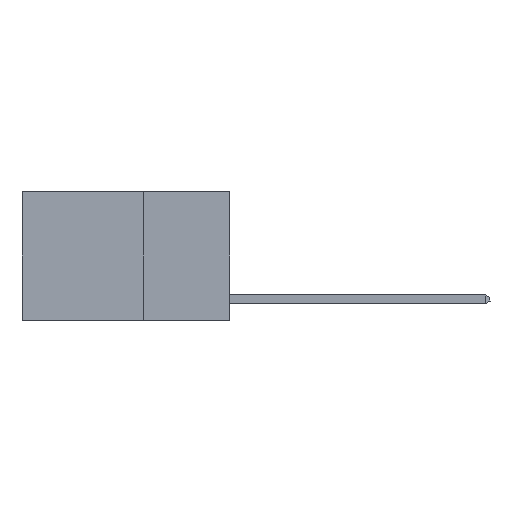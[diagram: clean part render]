
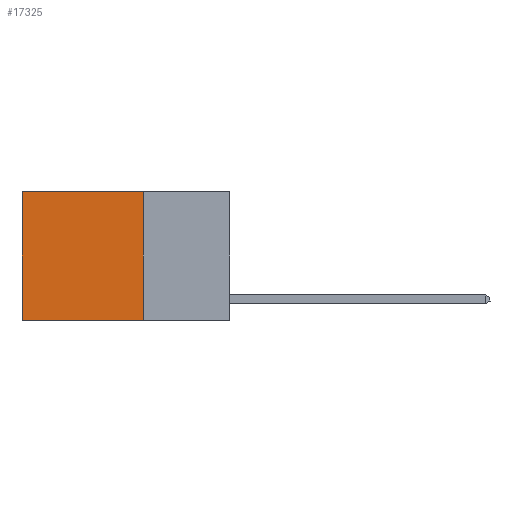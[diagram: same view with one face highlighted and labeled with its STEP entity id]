
A CAD part, left-side view. The second image highlights one B-rep face of the part: STEP entity #17325.
In plain terms, the highlighted planar face has unit normal (-1, 0, 0).
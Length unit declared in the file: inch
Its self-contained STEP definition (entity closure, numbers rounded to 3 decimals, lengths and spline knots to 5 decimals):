
#405 = DIRECTION ( 'NONE',  ( 0., 1., 0. ) ) ;
#759 = VERTEX_POINT ( 'NONE', #5656 ) ;
#1287 = VECTOR ( 'NONE', #2496, 39.37008 ) ;
#1519 = AXIS2_PLACEMENT_3D ( 'NONE', #7191, #17526, #19041 ) ;
#1536 = DIRECTION ( 'NONE',  ( 0., 0., -1. ) ) ;
#1639 = FACE_OUTER_BOUND ( 'NONE', #6550, .T. ) ;
#1722 = VERTEX_POINT ( 'NONE', #2591 ) ;
#1958 = LINE ( 'NONE', #14588, #13408 ) ;
#2084 = VERTEX_POINT ( 'NONE', #6615 ) ;
#2173 = EDGE_CURVE ( 'NONE', #759, #10164, #8049, .T. ) ;
#2398 = EDGE_CURVE ( 'NONE', #1722, #2084, #5228, .T. ) ;
#2496 = DIRECTION ( 'NONE',  ( 0., 1., 0. ) ) ;
#2591 = CARTESIAN_POINT ( 'NONE',  ( 0.2625, 0.25, 0. ) ) ;
#2771 = EDGE_CURVE ( 'NONE', #1722, #759, #1958, .T. ) ;
#3791 = ORIENTED_EDGE ( 'NONE', *, *, #2771, .F. ) ;
#5228 = LINE ( 'NONE', #18897, #1287 ) ;
#5656 = CARTESIAN_POINT ( 'NONE',  ( 0.2625, 0.25, -0.37 ) ) ;
#5849 = VECTOR ( 'NONE', #1536, 39.37008 ) ;
#6550 = EDGE_LOOP ( 'NONE', ( #8324, #12034, #3791, #16343 ) ) ;
#6615 = CARTESIAN_POINT ( 'NONE',  ( 0.2625, 0.6, 0. ) ) ;
#6883 = VECTOR ( 'NONE', #405, 39.37008 ) ;
#7125 = PLANE ( 'NONE',  #1519 ) ;
#7191 = CARTESIAN_POINT ( 'NONE',  ( 0.2625, 0.25, 0. ) ) ;
#7305 = CARTESIAN_POINT ( 'NONE',  ( 0.2625, 0.6, -0.37 ) ) ;
#8049 = LINE ( 'NONE', #16992, #6883 ) ;
#8324 = ORIENTED_EDGE ( 'NONE', *, *, #16949, .T. ) ;
#10164 = VERTEX_POINT ( 'NONE', #7305 ) ;
#12034 = ORIENTED_EDGE ( 'NONE', *, *, #2173, .F. ) ;
#13408 = VECTOR ( 'NONE', #19075, 39.37008 ) ;
#14588 = CARTESIAN_POINT ( 'NONE',  ( 0.2625, 0.25, 0. ) ) ;
#14888 = CARTESIAN_POINT ( 'NONE',  ( 0.2625, 0.6, 0. ) ) ;
#16343 = ORIENTED_EDGE ( 'NONE', *, *, #2398, .T. ) ;
#16949 = EDGE_CURVE ( 'NONE', #2084, #10164, #18653, .T. ) ;
#16992 = CARTESIAN_POINT ( 'NONE',  ( 0.2625, 0.25, -0.37 ) ) ;
#17325 = ADVANCED_FACE ( 'NONE', ( #1639 ), #7125, .F. ) ;
#17526 = DIRECTION ( 'NONE',  ( 1., 0., 0. ) ) ;
#18653 = LINE ( 'NONE', #14888, #5849 ) ;
#18897 = CARTESIAN_POINT ( 'NONE',  ( 0.2625, 0.25, 0. ) ) ;
#19041 = DIRECTION ( 'NONE',  ( 0., 0., -1. ) ) ;
#19075 = DIRECTION ( 'NONE',  ( 0., 0., -1. ) ) ;
